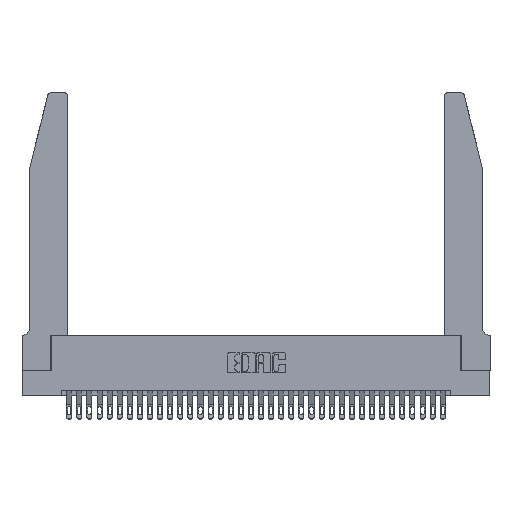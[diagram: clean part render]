
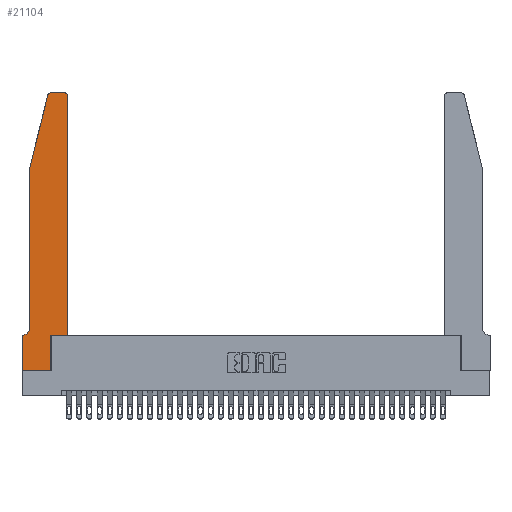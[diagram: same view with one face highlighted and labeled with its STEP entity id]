
A CAD part, top view. The second image highlights one B-rep face of the part: STEP entity #21104.
In plain terms, the highlighted planar face has unit normal (0, 0, 1).
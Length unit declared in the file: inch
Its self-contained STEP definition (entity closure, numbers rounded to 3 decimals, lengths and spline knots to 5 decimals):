
#93 = ORIENTED_EDGE ( 'NONE', *, *, #20085, .T. ) ;
#379 = CARTESIAN_POINT ( 'NONE',  ( 0.0055, 0.42, 0.37 ) ) ;
#566 = CARTESIAN_POINT ( 'NONE',  ( 0.4505, 0.35, 0.37 ) ) ;
#825 = CARTESIAN_POINT ( 'NONE',  ( 0.2605, 2.75, 0.37 ) ) ;
#1665 = CARTESIAN_POINT ( 'NONE',  ( 0.4505, 0.35, 0.37 ) ) ;
#1980 = VERTEX_POINT ( 'NONE', #11217 ) ;
#3873 = CARTESIAN_POINT ( 'NONE',  ( 0., 0., 0.37 ) ) ;
#3919 = VECTOR ( 'NONE', #28007, 39.37008 ) ;
#4391 = CARTESIAN_POINT ( 'NONE',  ( 0.2865, 0.35, 0.37 ) ) ;
#4607 = EDGE_CURVE ( 'NONE', #10383, #14570, #18279, .T. ) ;
#4995 = PLANE ( 'NONE',  #35087 ) ;
#5168 = CARTESIAN_POINT ( 'NONE',  ( 0.0755, 2., 0.37 ) ) ;
#5450 = AXIS2_PLACEMENT_3D ( 'NONE', #11438, #14424, #6076 ) ;
#6070 = VECTOR ( 'NONE', #6916, 39.37008 ) ;
#6076 = DIRECTION ( 'NONE',  ( 1., 0., 0. ) ) ;
#6241 = ORIENTED_EDGE ( 'NONE', *, *, #14893, .T. ) ;
#6916 = DIRECTION ( 'NONE',  ( 0., -1., 0. ) ) ;
#6941 = CARTESIAN_POINT ( 'NONE',  ( 0.0755, 0.35, 0.37 ) ) ;
#7299 = VECTOR ( 'NONE', #13463, 39.37008 ) ;
#7344 = EDGE_CURVE ( 'NONE', #11516, #31798, #13666, .T. ) ;
#8037 = CARTESIAN_POINT ( 'NONE',  ( 0.2865, 0., 0.37 ) ) ;
#8201 = DIRECTION ( 'NONE',  ( 0., 0., 1. ) ) ;
#8635 = DIRECTION ( 'NONE',  ( 0., 0., -1. ) ) ;
#9801 = CARTESIAN_POINT ( 'NONE',  ( 0.0755, 0.42, 0.37 ) ) ;
#10383 = VERTEX_POINT ( 'NONE', #5168 ) ;
#10402 = CARTESIAN_POINT ( 'NONE',  ( 0.4505, 2.72, 0.37 ) ) ;
#10722 = VERTEX_POINT ( 'NONE', #33373 ) ;
#10921 = LINE ( 'NONE', #1665, #14341 ) ;
#10940 = ORIENTED_EDGE ( 'NONE', *, *, #22969, .T. ) ;
#11172 = LINE ( 'NONE', #825, #3919 ) ;
#11217 = CARTESIAN_POINT ( 'NONE',  ( 0.25487, 2.72718, 0.37 ) ) ;
#11362 = DIRECTION ( 'NONE',  ( -1., 0., 0. ) ) ;
#11438 = CARTESIAN_POINT ( 'NONE',  ( 0.4205, 2.72, 0.37 ) ) ;
#11516 = VERTEX_POINT ( 'NONE', #25549 ) ;
#11750 = LINE ( 'NONE', #16964, #28482 ) ;
#12514 = CARTESIAN_POINT ( 'NONE',  ( 0., 0., 0.37 ) ) ;
#12870 = EDGE_CURVE ( 'NONE', #14570, #14514, #30563, .T. ) ;
#13063 = ORIENTED_EDGE ( 'NONE', *, *, #22261, .T. ) ;
#13463 = DIRECTION ( 'NONE',  ( 0., 1., 0. ) ) ;
#13666 = LINE ( 'NONE', #3873, #33027 ) ;
#13745 = ORIENTED_EDGE ( 'NONE', *, *, #12870, .T. ) ;
#14123 = LINE ( 'NONE', #16114, #7299 ) ;
#14341 = VECTOR ( 'NONE', #18068, 39.37008 ) ;
#14424 = DIRECTION ( 'NONE',  ( 0., 0., 1. ) ) ;
#14514 = VERTEX_POINT ( 'NONE', #28138 ) ;
#14570 = VERTEX_POINT ( 'NONE', #9801 ) ;
#14677 = DIRECTION ( 'NONE',  ( -0.239, -0.971, 0. ) ) ;
#14703 = FACE_OUTER_BOUND ( 'NONE', #16505, .T. ) ;
#14893 = EDGE_CURVE ( 'NONE', #23257, #22242, #25905, .T. ) ;
#16114 = CARTESIAN_POINT ( 'NONE',  ( 0.2865, 0.35, 0.37 ) ) ;
#16146 = VERTEX_POINT ( 'NONE', #34574 ) ;
#16505 = EDGE_LOOP ( 'NONE', ( #24257, #20010, #93, #34205, #13745, #20052, #13063, #31210, #10940, #6241, #28638, #31183 ) ) ;
#16964 = CARTESIAN_POINT ( 'NONE',  ( 0.0755, 2., 0.37 ) ) ;
#17039 = CIRCLE ( 'NONE', #5450, 0.03 ) ;
#17828 = DIRECTION ( 'NONE',  ( -1., 0., 0. ) ) ;
#17948 = DIRECTION ( 'NONE',  ( 1., 0., 0. ) ) ;
#18068 = DIRECTION ( 'NONE',  ( 0., 1., 0. ) ) ;
#18279 = LINE ( 'NONE', #29249, #34582 ) ;
#18610 = EDGE_CURVE ( 'NONE', #19758, #31005, #17039, .T. ) ;
#18614 = DIRECTION ( 'NONE',  ( 1., 0., 0. ) ) ;
#18621 = VECTOR ( 'NONE', #17948, 39.37008 ) ;
#18873 = DIRECTION ( 'NONE',  ( 1., 0., 0. ) ) ;
#19758 = VERTEX_POINT ( 'NONE', #10402 ) ;
#20010 = ORIENTED_EDGE ( 'NONE', *, *, #29368, .T. ) ;
#20052 = ORIENTED_EDGE ( 'NONE', *, *, #30471, .T. ) ;
#20085 = EDGE_CURVE ( 'NONE', #1980, #10383, #11750, .T. ) ;
#20232 = EDGE_CURVE ( 'NONE', #22242, #19758, #10921, .T. ) ;
#20265 = DIRECTION ( 'NONE',  ( 1., 0., 0. ) ) ;
#21104 = ADVANCED_FACE ( 'NONE', ( #14703 ), #4995, .T. ) ;
#21501 = DIRECTION ( 'NONE',  ( 0., 0., 1. ) ) ;
#22242 = VERTEX_POINT ( 'NONE', #33747 ) ;
#22261 = EDGE_CURVE ( 'NONE', #10722, #11516, #31809, .T. ) ;
#22969 = EDGE_CURVE ( 'NONE', #31798, #23257, #14123, .T. ) ;
#23257 = VERTEX_POINT ( 'NONE', #4391 ) ;
#24257 = ORIENTED_EDGE ( 'NONE', *, *, #34640, .T. ) ;
#24401 = AXIS2_PLACEMENT_3D ( 'NONE', #379, #8635, #11362 ) ;
#24522 = CARTESIAN_POINT ( 'NONE',  ( 0.284, 2.72, 0.37 ) ) ;
#25549 = CARTESIAN_POINT ( 'NONE',  ( 0., 0., 0.37 ) ) ;
#25905 = LINE ( 'NONE', #566, #18621 ) ;
#26981 = AXIS2_PLACEMENT_3D ( 'NONE', #24522, #8201, #18873 ) ;
#28007 = DIRECTION ( 'NONE',  ( -1., 0., 0. ) ) ;
#28138 = CARTESIAN_POINT ( 'NONE',  ( 0.0055, 0.35, 0.37 ) ) ;
#28482 = VECTOR ( 'NONE', #14677, 39.37008 ) ;
#28638 = ORIENTED_EDGE ( 'NONE', *, *, #20232, .T. ) ;
#28688 = VECTOR ( 'NONE', #17828, 39.37008 ) ;
#29249 = CARTESIAN_POINT ( 'NONE',  ( 0.0755, 2., 0.37 ) ) ;
#29368 = EDGE_CURVE ( 'NONE', #16146, #1980, #35247, .T. ) ;
#30026 = LINE ( 'NONE', #6941, #28688 ) ;
#30471 = EDGE_CURVE ( 'NONE', #14514, #10722, #30026, .T. ) ;
#30563 = CIRCLE ( 'NONE', #24401, 0.07 ) ;
#30992 = DIRECTION ( 'NONE',  ( 0., -1., 0. ) ) ;
#31005 = VERTEX_POINT ( 'NONE', #31081 ) ;
#31081 = CARTESIAN_POINT ( 'NONE',  ( 0.4205, 2.75, 0.37 ) ) ;
#31183 = ORIENTED_EDGE ( 'NONE', *, *, #18610, .T. ) ;
#31210 = ORIENTED_EDGE ( 'NONE', *, *, #7344, .T. ) ;
#31798 = VERTEX_POINT ( 'NONE', #8037 ) ;
#31809 = LINE ( 'NONE', #12514, #6070 ) ;
#33027 = VECTOR ( 'NONE', #20265, 39.37008 ) ;
#33373 = CARTESIAN_POINT ( 'NONE',  ( 0., 0.35, 0.37 ) ) ;
#33747 = CARTESIAN_POINT ( 'NONE',  ( 0.4505, 0.35, 0.37 ) ) ;
#34205 = ORIENTED_EDGE ( 'NONE', *, *, #4607, .T. ) ;
#34574 = CARTESIAN_POINT ( 'NONE',  ( 0.284, 2.75, 0.37 ) ) ;
#34582 = VECTOR ( 'NONE', #30992, 39.37008 ) ;
#34640 = EDGE_CURVE ( 'NONE', #31005, #16146, #11172, .T. ) ;
#35087 = AXIS2_PLACEMENT_3D ( 'NONE', #35384, #21501, #18614 ) ;
#35247 = CIRCLE ( 'NONE', #26981, 0.03 ) ;
#35384 = CARTESIAN_POINT ( 'NONE',  ( 0., 0.35, 0.37 ) ) ;
